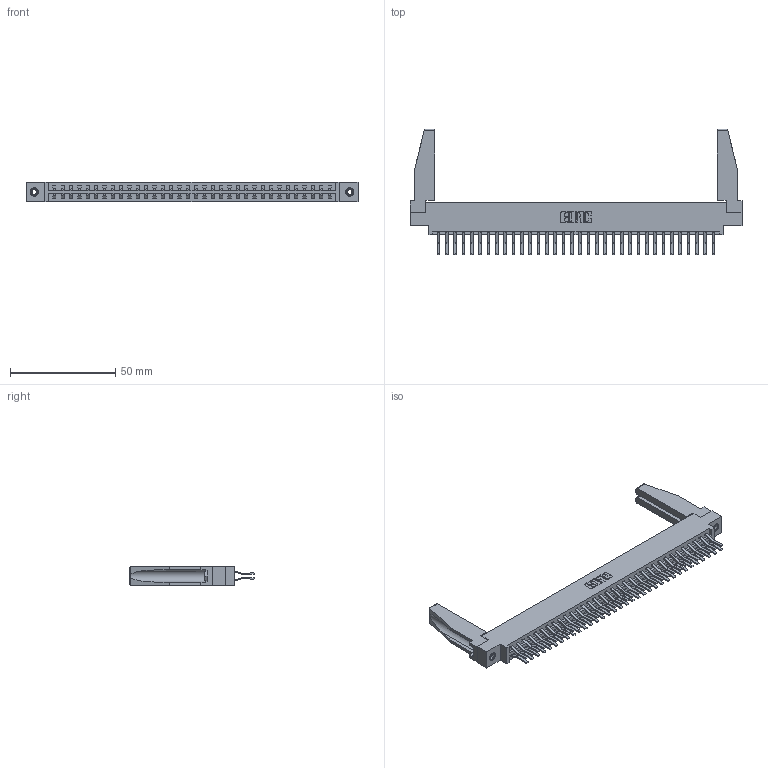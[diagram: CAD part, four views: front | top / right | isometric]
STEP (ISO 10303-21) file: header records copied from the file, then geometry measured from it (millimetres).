
FILE_DESCRIPTION (( 'STEP AP203' ), '1' );
FILE_NAME ('387-068-560-878.STEP', '2019-10-19T22:29:36', ( '' ), ( '' ), 'SwSTEP 2.0', 'SolidWorks 2016', '' );
FILE_SCHEMA (( 'CONFIG_CONTROL_DESIGN' ));
Length unit declared in the file: inch
Products named in the file (5): 307-220-078; 345-250-001_345-250-001-102; 337 Part_0.170 Offset - 0.156 Dia-TI; 345-292-001_560 Tail; 387-068-560-878
Assembly tree (73 placements, depth 2):
  387-068-560-878
    337 Part_0.170 Offset - 0.156 Dia-TI
    345-292-001_560 Tail  x68
    345-250-001_345-250-001-102  x2
    307-220-078  x2
Bounding box: 157.73 x 59.58 x 9.4 mm (x, y, z)
Volume: 20838.3 mm3; surface area: 24193.9 mm2
Topology: 73 solids, 73 shells, 4056 faces, 12009 edges, 7906 vertices
Faces by surface type: plane 2742, cylinder 1298, cone 12, torus 4
Entity records: 30056 total; most frequent: CARTESIAN_POINT 5072, ORIENTED_EDGE 4964, DIRECTION 4338, EDGE_CURVE 2482, LINE 2312, VECTOR 2312, VERTEX_POINT 1648, AXIS2_PLACEMENT_3D 1013
